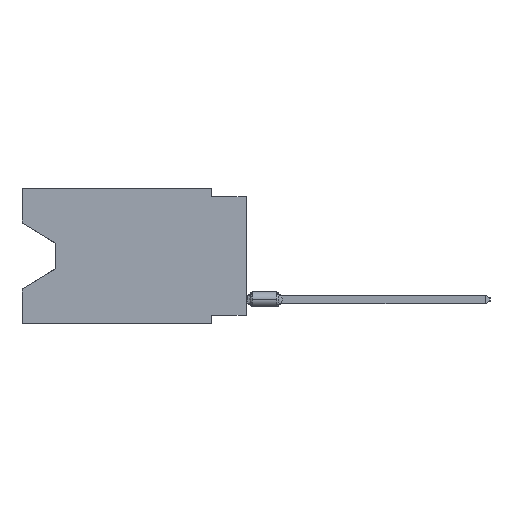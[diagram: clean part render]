
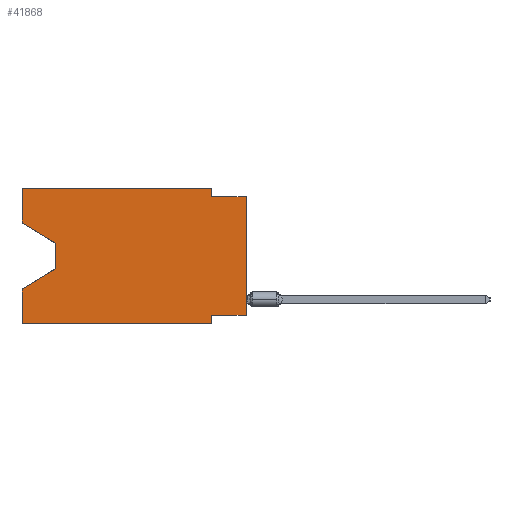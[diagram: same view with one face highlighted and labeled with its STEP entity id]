
A CAD part, left-side view. The second image highlights one B-rep face of the part: STEP entity #41868.
In plain terms, the highlighted planar face has unit normal (-1, 0, 0).
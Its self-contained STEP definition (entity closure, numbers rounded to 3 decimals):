
#206 = DIRECTION ( 'NONE',  ( 0., 1., 0. ) ) ;
#796 = VERTEX_POINT ( 'NONE', #3681 ) ;
#1466 = EDGE_CURVE ( 'NONE', #37359, #50940, #61080, .T. ) ;
#2062 = CARTESIAN_POINT ( 'NONE',  ( 0., 16.383, -2.546 ) ) ;
#2433 = VERTEX_POINT ( 'NONE', #42010 ) ;
#2448 = LINE ( 'NONE', #60194, #57529 ) ;
#3066 = VERTEX_POINT ( 'NONE', #12368 ) ;
#3436 = ORIENTED_EDGE ( 'NONE', *, *, #15102, .F. ) ;
#3681 = CARTESIAN_POINT ( 'NONE',  ( 0., 16.383, -9.906 ) ) ;
#5964 = DIRECTION ( 'NONE',  ( 0., -0.855, -0.519 ) ) ;
#6131 = LINE ( 'NONE', #42674, #66386 ) ;
#6823 = ORIENTED_EDGE ( 'NONE', *, *, #7404, .F. ) ;
#6873 = DIRECTION ( 'NONE',  ( 0., 0., 1. ) ) ;
#7404 = EDGE_CURVE ( 'NONE', #20449, #16432, #41597, .T. ) ;
#7780 = ORIENTED_EDGE ( 'NONE', *, *, #11733, .T. ) ;
#7903 = CARTESIAN_POINT ( 'NONE',  ( 0., 16.383, 0. ) ) ;
#8258 = ORIENTED_EDGE ( 'NONE', *, *, #17042, .F. ) ;
#9010 = EDGE_CURVE ( 'NONE', #33380, #22632, #64821, .T. ) ;
#9421 = CARTESIAN_POINT ( 'NONE',  ( 0., 0., -0.635 ) ) ;
#11098 = EDGE_CURVE ( 'NONE', #16432, #33380, #54703, .T. ) ;
#11733 = EDGE_CURVE ( 'NONE', #20449, #37359, #45618, .T. ) ;
#12050 = DIRECTION ( 'NONE',  ( 0., 0., 1. ) ) ;
#12368 = CARTESIAN_POINT ( 'NONE',  ( 0., 2.54, -9.271 ) ) ;
#13982 = DIRECTION ( 'NONE',  ( 0., 0., -1. ) ) ;
#15102 = EDGE_CURVE ( 'NONE', #3066, #36005, #29917, .T. ) ;
#15171 = CARTESIAN_POINT ( 'NONE',  ( 0., 2.54, -0.635 ) ) ;
#15290 = LINE ( 'NONE', #31985, #66000 ) ;
#15655 = DIRECTION ( 'NONE',  ( 0., 0., 1. ) ) ;
#16356 = VECTOR ( 'NONE', #46309, 1000. ) ;
#16432 = VERTEX_POINT ( 'NONE', #38194 ) ;
#17042 = EDGE_CURVE ( 'NONE', #796, #2433, #37955, .T. ) ;
#17490 = CARTESIAN_POINT ( 'NONE',  ( 0., 2.54, -9.906 ) ) ;
#18512 = EDGE_CURVE ( 'NONE', #22632, #54993, #60950, .T. ) ;
#18785 = EDGE_CURVE ( 'NONE', #66509, #54993, #2448, .T. ) ;
#20004 = CARTESIAN_POINT ( 'NONE',  ( 0., 2.54, -9.906 ) ) ;
#20449 = VERTEX_POINT ( 'NONE', #2062 ) ;
#20895 = CARTESIAN_POINT ( 'NONE',  ( 0., 16.383, 0. ) ) ;
#21456 = CARTESIAN_POINT ( 'NONE',  ( 0., 13.97, -5.893 ) ) ;
#22632 = VERTEX_POINT ( 'NONE', #15171 ) ;
#23842 = DIRECTION ( 'NONE',  ( 0., 0., -1. ) ) ;
#24911 = AXIS2_PLACEMENT_3D ( 'NONE', #39945, #60799, #13982 ) ;
#26737 = ORIENTED_EDGE ( 'NONE', *, *, #46275, .T. ) ;
#28433 = VECTOR ( 'NONE', #36146, 1000. ) ;
#29897 = VECTOR ( 'NONE', #15655, 1000. ) ;
#29917 = LINE ( 'NONE', #20004, #16356 ) ;
#31985 = CARTESIAN_POINT ( 'NONE',  ( 0., 0., -9.271 ) ) ;
#32101 = CARTESIAN_POINT ( 'NONE',  ( 0., 2.54, 0. ) ) ;
#33380 = VERTEX_POINT ( 'NONE', #32101 ) ;
#33518 = DIRECTION ( 'NONE',  ( 0., -1., 0. ) ) ;
#34018 = DIRECTION ( 'NONE',  ( 0., 0., -1. ) ) ;
#34308 = ORIENTED_EDGE ( 'NONE', *, *, #9010, .F. ) ;
#34680 = ORIENTED_EDGE ( 'NONE', *, *, #11098, .F. ) ;
#34708 = CARTESIAN_POINT ( 'NONE',  ( 0., 13.97, -5.893 ) ) ;
#35448 = ORIENTED_EDGE ( 'NONE', *, *, #36713, .F. ) ;
#35584 = VECTOR ( 'NONE', #5964, 1000. ) ;
#36005 = VERTEX_POINT ( 'NONE', #17490 ) ;
#36146 = DIRECTION ( 'NONE',  ( 0., 0.855, -0.519 ) ) ;
#36713 = EDGE_CURVE ( 'NONE', #66509, #3066, #15290, .T. ) ;
#37359 = VERTEX_POINT ( 'NONE', #51238 ) ;
#37955 = LINE ( 'NONE', #20895, #50207 ) ;
#38194 = CARTESIAN_POINT ( 'NONE',  ( 0., 16.383, 0. ) ) ;
#39945 = CARTESIAN_POINT ( 'NONE',  ( 0., 16.383, 0. ) ) ;
#40158 = VECTOR ( 'NONE', #23842, 1000. ) ;
#40949 = LINE ( 'NONE', #21456, #28433 ) ;
#41597 = LINE ( 'NONE', #62450, #29897 ) ;
#41868 = ADVANCED_FACE ( 'NONE', ( #66946 ), #50517, .F. ) ;
#42010 = CARTESIAN_POINT ( 'NONE',  ( 0., 16.383, -7.36 ) ) ;
#42674 = CARTESIAN_POINT ( 'NONE',  ( 0., 16.383, -9.906 ) ) ;
#42682 = ORIENTED_EDGE ( 'NONE', *, *, #67098, .T. ) ;
#45618 = LINE ( 'NONE', #58917, #35584 ) ;
#45875 = CARTESIAN_POINT ( 'NONE',  ( 0., 0., -9.271 ) ) ;
#46275 = EDGE_CURVE ( 'NONE', #50940, #2433, #40949, .T. ) ;
#46309 = DIRECTION ( 'NONE',  ( 0., 0., -1. ) ) ;
#47797 = DIRECTION ( 'NONE',  ( 0., -1., 0. ) ) ;
#49125 = ORIENTED_EDGE ( 'NONE', *, *, #18785, .T. ) ;
#49538 = ORIENTED_EDGE ( 'NONE', *, *, #18512, .F. ) ;
#50207 = VECTOR ( 'NONE', #6873, 1000. ) ;
#50517 = PLANE ( 'NONE',  #24911 ) ;
#50818 = VECTOR ( 'NONE', #56831, 1000. ) ;
#50940 = VERTEX_POINT ( 'NONE', #34708 ) ;
#51238 = CARTESIAN_POINT ( 'NONE',  ( 0., 13.97, -4.013 ) ) ;
#54686 = ORIENTED_EDGE ( 'NONE', *, *, #1466, .T. ) ;
#54703 = LINE ( 'NONE', #7903, #66093 ) ;
#54878 = CARTESIAN_POINT ( 'NONE',  ( 0., 2.54, 0. ) ) ;
#54993 = VERTEX_POINT ( 'NONE', #9421 ) ;
#55946 = CARTESIAN_POINT ( 'NONE',  ( 0., 13.97, -4.013 ) ) ;
#56022 = VECTOR ( 'NONE', #34018, 1000. ) ;
#56831 = DIRECTION ( 'NONE',  ( 0., -1., 0. ) ) ;
#57529 = VECTOR ( 'NONE', #12050, 1000. ) ;
#58917 = CARTESIAN_POINT ( 'NONE',  ( 0., 16.383, -2.546 ) ) ;
#60194 = CARTESIAN_POINT ( 'NONE',  ( 0., 0., 0. ) ) ;
#60799 = DIRECTION ( 'NONE',  ( 1., 0., 0. ) ) ;
#60950 = LINE ( 'NONE', #65758, #50818 ) ;
#61080 = LINE ( 'NONE', #55946, #40158 ) ;
#62450 = CARTESIAN_POINT ( 'NONE',  ( 0., 16.383, 0. ) ) ;
#64821 = LINE ( 'NONE', #54878, #56022 ) ;
#64988 = EDGE_LOOP ( 'NONE', ( #7780, #54686, #26737, #8258, #42682, #3436, #35448, #49125, #49538, #34308, #34680, #6823 ) ) ;
#65758 = CARTESIAN_POINT ( 'NONE',  ( 0., 0., -0.635 ) ) ;
#66000 = VECTOR ( 'NONE', #206, 1000. ) ;
#66093 = VECTOR ( 'NONE', #33518, 1000. ) ;
#66386 = VECTOR ( 'NONE', #47797, 1000. ) ;
#66509 = VERTEX_POINT ( 'NONE', #45875 ) ;
#66946 = FACE_OUTER_BOUND ( 'NONE', #64988, .T. ) ;
#67098 = EDGE_CURVE ( 'NONE', #796, #36005, #6131, .T. ) ;
